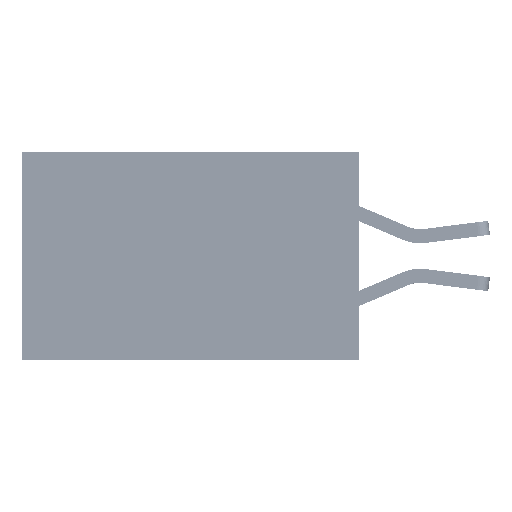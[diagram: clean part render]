
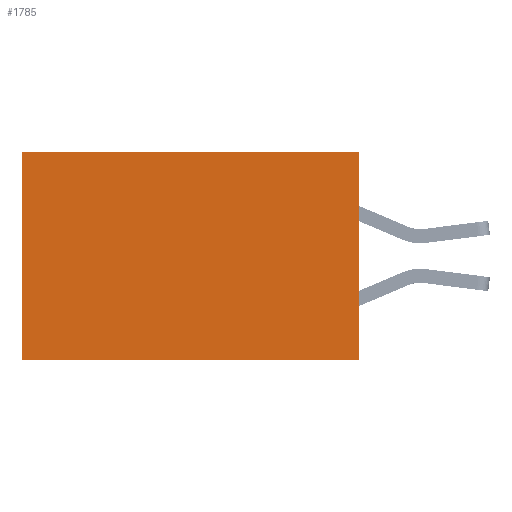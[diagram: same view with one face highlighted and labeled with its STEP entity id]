
A CAD part, left-side view. The second image highlights one B-rep face of the part: STEP entity #1785.
In plain terms, the highlighted planar face has unit normal (-1, 0, 0).
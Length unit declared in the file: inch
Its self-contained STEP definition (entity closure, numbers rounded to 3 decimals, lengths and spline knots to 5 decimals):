
#1785 = ADVANCED_FACE ( 'NONE', ( #2532 ), #38559, .F. ) ;
#2532 = FACE_OUTER_BOUND ( 'NONE', #21986, .T. ) ;
#3566 = CARTESIAN_POINT ( 'NONE',  ( 0.2875, 0.6, -0.37 ) ) ;
#4334 = CARTESIAN_POINT ( 'NONE',  ( 0.2875, 0., 0. ) ) ;
#5845 = DIRECTION ( 'NONE',  ( 0., 0., -1. ) ) ;
#7118 = CARTESIAN_POINT ( 'NONE',  ( 0.2875, 0., -0.37 ) ) ;
#8458 = VERTEX_POINT ( 'NONE', #3566 ) ;
#9523 = VECTOR ( 'NONE', #5845, 39.37008 ) ;
#11148 = ORIENTED_EDGE ( 'NONE', *, *, #18119, .F. ) ;
#11685 = DIRECTION ( 'NONE',  ( 0., 1., 0. ) ) ;
#15763 = VECTOR ( 'NONE', #29185, 39.37008 ) ;
#16978 = DIRECTION ( 'NONE',  ( 1., 0., 0. ) ) ;
#17998 = CARTESIAN_POINT ( 'NONE',  ( 0.2875, 0., -0.37 ) ) ;
#18119 = EDGE_CURVE ( 'NONE', #18144, #8458, #20902, .T. ) ;
#18144 = VERTEX_POINT ( 'NONE', #7118 ) ;
#20612 = CARTESIAN_POINT ( 'NONE',  ( 0.2875, 0., 0. ) ) ;
#20676 = DIRECTION ( 'NONE',  ( 0., 0., -1. ) ) ;
#20902 = LINE ( 'NONE', #17998, #15763 ) ;
#21986 = EDGE_LOOP ( 'NONE', ( #40925, #11148, #44546, #37977 ) ) ;
#22024 = LINE ( 'NONE', #4334, #24874 ) ;
#23142 = EDGE_CURVE ( 'NONE', #29360, #18144, #35227, .T. ) ;
#24121 = EDGE_CURVE ( 'NONE', #29360, #29925, #22024, .T. ) ;
#24727 = LINE ( 'NONE', #44913, #37868 ) ;
#24874 = VECTOR ( 'NONE', #11685, 39.37008 ) ;
#26050 = CARTESIAN_POINT ( 'NONE',  ( 0.2875, 0.6, 0. ) ) ;
#27900 = CARTESIAN_POINT ( 'NONE',  ( 0.2875, 0., 0. ) ) ;
#29185 = DIRECTION ( 'NONE',  ( 0., 1., 0. ) ) ;
#29360 = VERTEX_POINT ( 'NONE', #20612 ) ;
#29925 = VERTEX_POINT ( 'NONE', #26050 ) ;
#31200 = EDGE_CURVE ( 'NONE', #29925, #8458, #24727, .T. ) ;
#31488 = AXIS2_PLACEMENT_3D ( 'NONE', #35336, #16978, #20676 ) ;
#35227 = LINE ( 'NONE', #27900, #9523 ) ;
#35336 = CARTESIAN_POINT ( 'NONE',  ( 0.2875, 0., 0. ) ) ;
#37868 = VECTOR ( 'NONE', #45059, 39.37008 ) ;
#37977 = ORIENTED_EDGE ( 'NONE', *, *, #24121, .T. ) ;
#38559 = PLANE ( 'NONE',  #31488 ) ;
#40925 = ORIENTED_EDGE ( 'NONE', *, *, #31200, .T. ) ;
#44546 = ORIENTED_EDGE ( 'NONE', *, *, #23142, .F. ) ;
#44913 = CARTESIAN_POINT ( 'NONE',  ( 0.2875, 0.6, 0. ) ) ;
#45059 = DIRECTION ( 'NONE',  ( 0., 0., -1. ) ) ;
